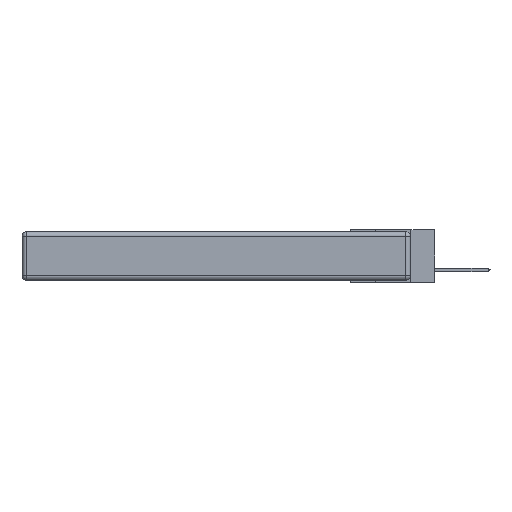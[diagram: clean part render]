
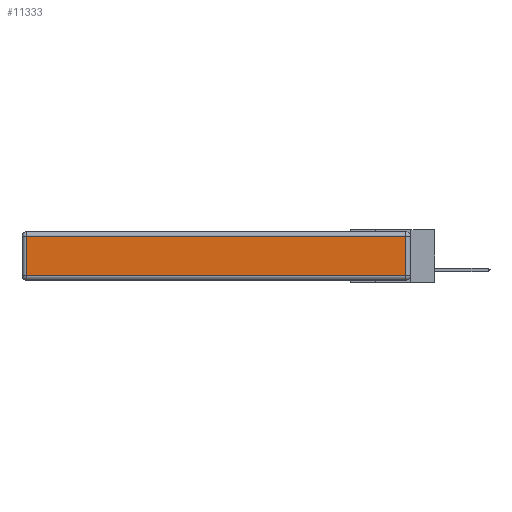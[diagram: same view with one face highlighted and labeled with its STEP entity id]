
A CAD part, left-side view. The second image highlights one B-rep face of the part: STEP entity #11333.
In plain terms, the highlighted planar face has unit normal (-1, 0, 0).
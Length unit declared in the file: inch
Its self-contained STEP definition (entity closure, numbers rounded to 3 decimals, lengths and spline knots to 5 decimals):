
#107 = EDGE_CURVE ( 'NONE', #4369, #11073, #8375, .T. ) ;
#1694 = LINE ( 'NONE', #13085, #12085 ) ;
#2156 = VECTOR ( 'NONE', #6948, 39.37008 ) ;
#2586 = DIRECTION ( 'NONE',  ( 0., 1., 0. ) ) ;
#3576 = VERTEX_POINT ( 'NONE', #9208 ) ;
#3578 = ORIENTED_EDGE ( 'NONE', *, *, #6089, .T. ) ;
#3607 = ORIENTED_EDGE ( 'NONE', *, *, #107, .T. ) ;
#3854 = DIRECTION ( 'NONE',  ( 0., 0., 1. ) ) ;
#3917 = DIRECTION ( 'NONE',  ( 0., 0., 1. ) ) ;
#3947 = CARTESIAN_POINT ( 'NONE',  ( 0., 0.03, -0.343 ) ) ;
#4369 = VERTEX_POINT ( 'NONE', #6124 ) ;
#4449 = CARTESIAN_POINT ( 'NONE',  ( 0., 2.72, -0.03 ) ) ;
#5504 = LINE ( 'NONE', #3947, #12987 ) ;
#6089 = EDGE_CURVE ( 'NONE', #11073, #3576, #5504, .T. ) ;
#6124 = CARTESIAN_POINT ( 'NONE',  ( 0., 2.72, -0.313 ) ) ;
#6948 = DIRECTION ( 'NONE',  ( 0., -1., 0. ) ) ;
#7018 = ORIENTED_EDGE ( 'NONE', *, *, #11754, .T. ) ;
#7206 = FACE_OUTER_BOUND ( 'NONE', #11075, .T. ) ;
#8020 = CARTESIAN_POINT ( 'NONE',  ( 0., 0., -0.313 ) ) ;
#8129 = CARTESIAN_POINT ( 'NONE',  ( 0., 0.03, -0.313 ) ) ;
#8375 = LINE ( 'NONE', #8020, #2156 ) ;
#9208 = CARTESIAN_POINT ( 'NONE',  ( 0., 0.03, -0.03 ) ) ;
#9212 = VERTEX_POINT ( 'NONE', #4449 ) ;
#10320 = AXIS2_PLACEMENT_3D ( 'NONE', #14465, #12037, #3917 ) ;
#10480 = VECTOR ( 'NONE', #2586, 39.37008 ) ;
#11073 = VERTEX_POINT ( 'NONE', #8129 ) ;
#11075 = EDGE_LOOP ( 'NONE', ( #3607, #3578, #7018, #12500 ) ) ;
#11333 = ADVANCED_FACE ( 'NONE', ( #7206 ), #12168, .T. ) ;
#11754 = EDGE_CURVE ( 'NONE', #3576, #9212, #13930, .T. ) ;
#12037 = DIRECTION ( 'NONE',  ( -1., 0., 0. ) ) ;
#12085 = VECTOR ( 'NONE', #13035, 39.37008 ) ;
#12154 = EDGE_CURVE ( 'NONE', #9212, #4369, #1694, .T. ) ;
#12168 = PLANE ( 'NONE',  #10320 ) ;
#12500 = ORIENTED_EDGE ( 'NONE', *, *, #12154, .T. ) ;
#12987 = VECTOR ( 'NONE', #3854, 39.37008 ) ;
#13035 = DIRECTION ( 'NONE',  ( 0., 0., -1. ) ) ;
#13085 = CARTESIAN_POINT ( 'NONE',  ( 0., 2.72, -0.343 ) ) ;
#13257 = CARTESIAN_POINT ( 'NONE',  ( 0., 2.75, -0.03 ) ) ;
#13930 = LINE ( 'NONE', #13257, #10480 ) ;
#14465 = CARTESIAN_POINT ( 'NONE',  ( 0., 0., -0.343 ) ) ;
